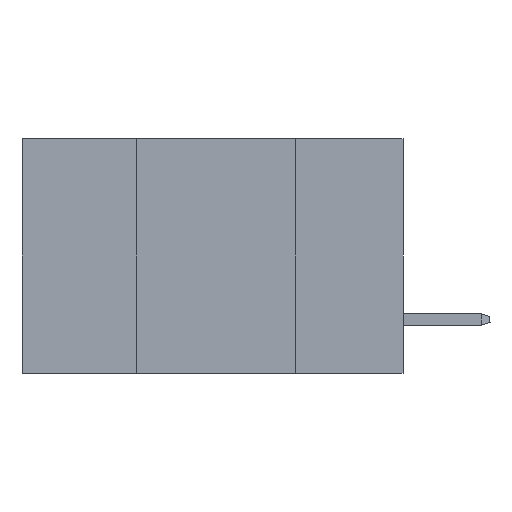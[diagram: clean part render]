
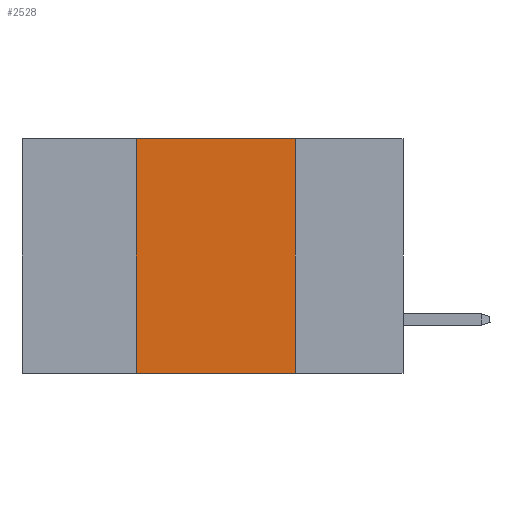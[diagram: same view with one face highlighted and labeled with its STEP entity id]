
A CAD part, left-side view. The second image highlights one B-rep face of the part: STEP entity #2528.
In plain terms, the highlighted planar face has unit normal (-1, 0, 0).
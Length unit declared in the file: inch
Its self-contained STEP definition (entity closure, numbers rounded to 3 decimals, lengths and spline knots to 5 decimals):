
#2528 = ADVANCED_FACE ( 'NONE', ( #22903 ), #7310, .F. ) ;
#2834 = CARTESIAN_POINT ( 'NONE',  ( 0., 0.6, -0.37 ) ) ;
#3402 = ORIENTED_EDGE ( 'NONE', *, *, #31241, .F. ) ;
#3991 = VERTEX_POINT ( 'NONE', #14897 ) ;
#5324 = VECTOR ( 'NONE', #25604, 39.37008 ) ;
#5639 = ORIENTED_EDGE ( 'NONE', *, *, #20516, .T. ) ;
#6160 = VECTOR ( 'NONE', #18012, 39.37008 ) ;
#7310 = PLANE ( 'NONE',  #15611 ) ;
#7694 = LINE ( 'NONE', #24541, #6160 ) ;
#8987 = LINE ( 'NONE', #34692, #37601 ) ;
#14897 = CARTESIAN_POINT ( 'NONE',  ( 0., 0.17, -0.37 ) ) ;
#15051 = VECTOR ( 'NONE', #26939, 39.37008 ) ;
#15611 = AXIS2_PLACEMENT_3D ( 'NONE', #33241, #35751, #17014 ) ;
#17014 = DIRECTION ( 'NONE',  ( 0., 0., -1. ) ) ;
#17033 = VERTEX_POINT ( 'NONE', #28587 ) ;
#18012 = DIRECTION ( 'NONE',  ( 0., 0., 1. ) ) ;
#18461 = LINE ( 'NONE', #2834, #5324 ) ;
#20516 = EDGE_CURVE ( 'NONE', #23253, #3991, #18461, .T. ) ;
#22903 = FACE_OUTER_BOUND ( 'NONE', #27610, .T. ) ;
#22943 = LINE ( 'NONE', #26734, #15051 ) ;
#23253 = VERTEX_POINT ( 'NONE', #37522 ) ;
#24541 = CARTESIAN_POINT ( 'NONE',  ( 0., 0.42, 0. ) ) ;
#24799 = ORIENTED_EDGE ( 'NONE', *, *, #38745, .F. ) ;
#25604 = DIRECTION ( 'NONE',  ( 0., -1., 0. ) ) ;
#26734 = CARTESIAN_POINT ( 'NONE',  ( 0., 0.17, 0. ) ) ;
#26939 = DIRECTION ( 'NONE',  ( 0., 0., -1. ) ) ;
#27610 = EDGE_LOOP ( 'NONE', ( #24799, #3402, #36685, #5639 ) ) ;
#28587 = CARTESIAN_POINT ( 'NONE',  ( 0., 0.17, 0. ) ) ;
#30931 = DIRECTION ( 'NONE',  ( 0., -1., 0. ) ) ;
#31241 = EDGE_CURVE ( 'NONE', #32079, #17033, #8987, .T. ) ;
#32079 = VERTEX_POINT ( 'NONE', #36739 ) ;
#33241 = CARTESIAN_POINT ( 'NONE',  ( 0., 0.6, 0. ) ) ;
#34692 = CARTESIAN_POINT ( 'NONE',  ( 0., 0.6, 0. ) ) ;
#34945 = EDGE_CURVE ( 'NONE', #23253, #32079, #7694, .T. ) ;
#35751 = DIRECTION ( 'NONE',  ( 1., 0., 0. ) ) ;
#36685 = ORIENTED_EDGE ( 'NONE', *, *, #34945, .F. ) ;
#36739 = CARTESIAN_POINT ( 'NONE',  ( 0., 0.42, 0. ) ) ;
#37522 = CARTESIAN_POINT ( 'NONE',  ( 0., 0.42, -0.37 ) ) ;
#37601 = VECTOR ( 'NONE', #30931, 39.37008 ) ;
#38745 = EDGE_CURVE ( 'NONE', #17033, #3991, #22943, .T. ) ;
